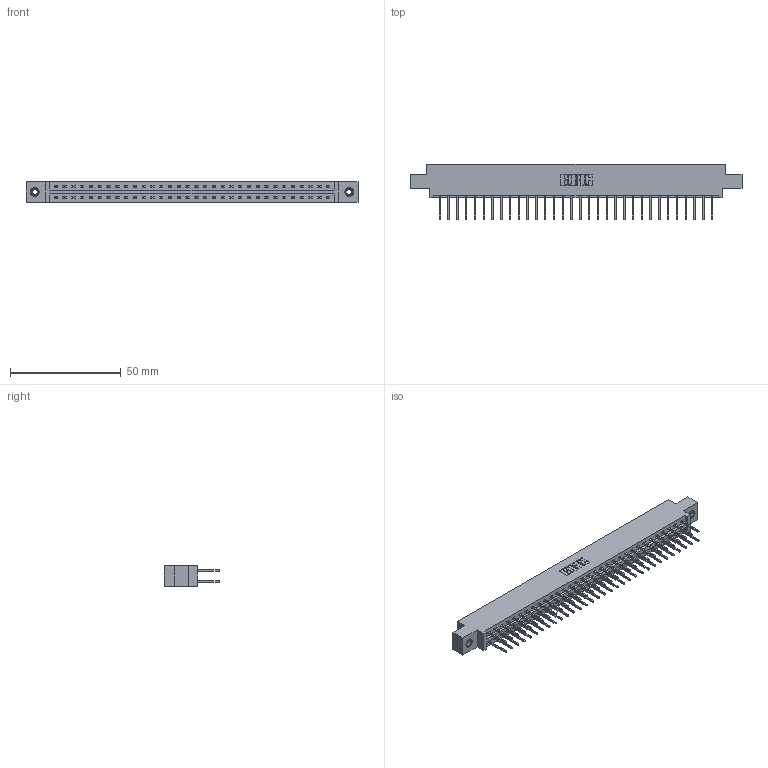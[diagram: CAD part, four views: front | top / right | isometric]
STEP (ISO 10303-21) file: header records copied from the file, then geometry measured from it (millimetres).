
FILE_DESCRIPTION (( 'STEP AP203' ), '1' );
FILE_NAME ('337-064-523-808.STEP', '2019-10-11T23:36:12', ( '' ), ( '' ), 'SwSTEP 2.0', 'SolidWorks 2016', '' );
FILE_SCHEMA (( 'CONFIG_CONTROL_DESIGN' ));
Length unit declared in the file: inch
Products named in the file (4): 337-064-523-808; 337 Part_0.170 Offset - 0.156 Dia-TI; 345-292-001_345-293-123; 345-250-001_345-250-003-102
Assembly tree (67 placements, depth 2):
  337-064-523-808
    337 Part_0.170 Offset - 0.156 Dia-TI
    345-292-001_345-293-123  x64
    345-250-001_345-250-003-102  x2
Bounding box: 149.81 x 25.15 x 9.4 mm (x, y, z)
Volume: 15662.1 mm3; surface area: 18364.1 mm2
Topology: 67 solids, 67 shells, 3634 faces, 10763 edges, 7082 vertices
Faces by surface type: plane 2538, cylinder 1080, cone 12, torus 4
Entity records: 27440 total; most frequent: CARTESIAN_POINT 4613, ORIENTED_EDGE 4542, DIRECTION 3973, EDGE_CURVE 2271, LINE 2123, VECTOR 2123, VERTEX_POINT 1508, AXIS2_PLACEMENT_3D 925
